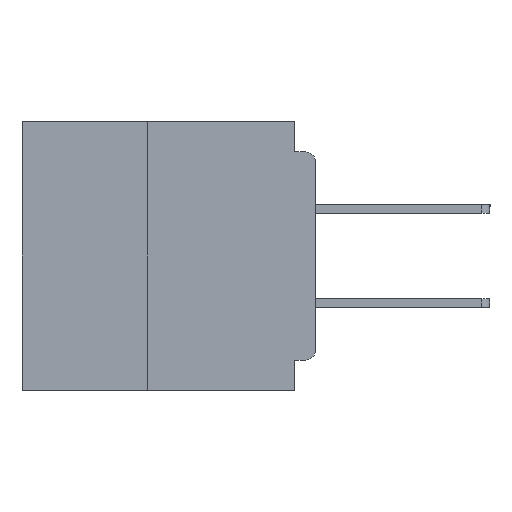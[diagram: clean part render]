
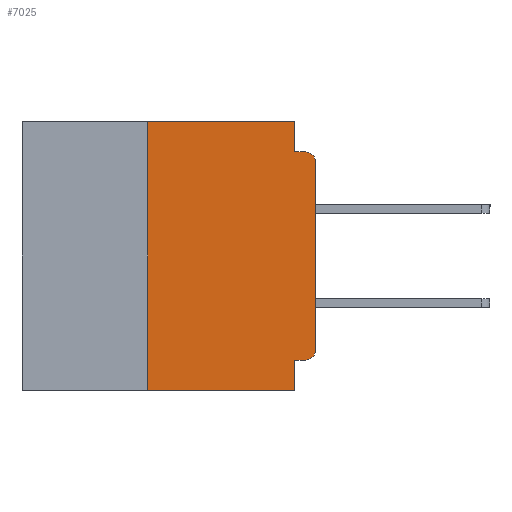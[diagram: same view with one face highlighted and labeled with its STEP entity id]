
A CAD part, left-side view. The second image highlights one B-rep face of the part: STEP entity #7025.
In plain terms, the highlighted planar face has unit normal (-1, 0, 0).
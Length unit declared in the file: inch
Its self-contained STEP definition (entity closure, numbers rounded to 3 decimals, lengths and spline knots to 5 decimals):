
#572 = CARTESIAN_POINT ( 'NONE',  ( 0., 0.25, -0.4 ) ) ;
#629 = VERTEX_POINT ( 'NONE', #41840 ) ;
#708 = EDGE_CURVE ( 'NONE', #14228, #19396, #25253, .T. ) ;
#2983 = VERTEX_POINT ( 'NONE', #5823 ) ;
#3160 = ORIENTED_EDGE ( 'NONE', *, *, #9187, .F. ) ;
#3955 = VECTOR ( 'NONE', #57200, 39.37008 ) ;
#4021 = CARTESIAN_POINT ( 'NONE',  ( 0., 0.031, 0. ) ) ;
#4068 = LINE ( 'NONE', #31584, #53552 ) ;
#4094 = FACE_OUTER_BOUND ( 'NONE', #14544, .T. ) ;
#4369 = DIRECTION ( 'NONE',  ( 0., 0., -1. ) ) ;
#4866 = CARTESIAN_POINT ( 'NONE',  ( 0., 0.25, 0. ) ) ;
#4978 = CARTESIAN_POINT ( 'NONE',  ( 0., 0.031, -0.4 ) ) ;
#5363 = ORIENTED_EDGE ( 'NONE', *, *, #708, .F. ) ;
#5823 = CARTESIAN_POINT ( 'NONE',  ( 0., 0.031, 0. ) ) ;
#7025 = ADVANCED_FACE ( 'NONE', ( #4094 ), #35545, .F. ) ;
#7192 = ORIENTED_EDGE ( 'NONE', *, *, #42871, .F. ) ;
#7927 = EDGE_CURVE ( 'NONE', #8041, #629, #40062, .T. ) ;
#8041 = VERTEX_POINT ( 'NONE', #54404 ) ;
#8421 = AXIS2_PLACEMENT_3D ( 'NONE', #27969, #61461, #32789 ) ;
#9187 = EDGE_CURVE ( 'NONE', #36276, #23664, #55641, .T. ) ;
#9914 = CARTESIAN_POINT ( 'NONE',  ( 0., 0.015, -0.045 ) ) ;
#10150 = EDGE_CURVE ( 'NONE', #22736, #23664, #25517, .T. ) ;
#10203 = DIRECTION ( 'NONE',  ( 0., 0., 1. ) ) ;
#11005 = VECTOR ( 'NONE', #36324, 39.37008 ) ;
#11325 = ORIENTED_EDGE ( 'NONE', *, *, #7927, .T. ) ;
#13453 = VERTEX_POINT ( 'NONE', #34746 ) ;
#14228 = VERTEX_POINT ( 'NONE', #31449 ) ;
#14544 = EDGE_LOOP ( 'NONE', ( #39849, #36387, #3160, #15448, #15174, #7192, #41543, #5363, #51667, #11325 ) ) ;
#15174 = ORIENTED_EDGE ( 'NONE', *, *, #57435, .F. ) ;
#15314 = CARTESIAN_POINT ( 'NONE',  ( 0., 0., -0.045 ) ) ;
#15448 = ORIENTED_EDGE ( 'NONE', *, *, #52084, .F. ) ;
#17462 = LINE ( 'NONE', #572, #27146 ) ;
#18926 = CARTESIAN_POINT ( 'NONE',  ( 0., 0., 0. ) ) ;
#19396 = VERTEX_POINT ( 'NONE', #33684 ) ;
#20051 = DIRECTION ( 'NONE',  ( -1., 0., 0. ) ) ;
#21300 = DIRECTION ( 'NONE',  ( 0., 0., -1. ) ) ;
#22736 = VERTEX_POINT ( 'NONE', #36203 ) ;
#23620 = LINE ( 'NONE', #43675, #58829 ) ;
#23664 = VERTEX_POINT ( 'NONE', #9914 ) ;
#23716 = LINE ( 'NONE', #55398, #11005 ) ;
#25253 = LINE ( 'NONE', #4978, #49271 ) ;
#25517 = CIRCLE ( 'NONE', #8421, 0.015 ) ;
#27146 = VECTOR ( 'NONE', #10203, 39.37008 ) ;
#27969 = CARTESIAN_POINT ( 'NONE',  ( 0., 0.015, -0.06 ) ) ;
#29386 = EDGE_CURVE ( 'NONE', #13453, #19396, #23620, .T. ) ;
#30171 = VECTOR ( 'NONE', #37528, 39.37008 ) ;
#30730 = CARTESIAN_POINT ( 'NONE',  ( 0., 0.437, 0. ) ) ;
#30935 = LINE ( 'NONE', #18926, #3955 ) ;
#31449 = CARTESIAN_POINT ( 'NONE',  ( 0., 0.031, -0.355 ) ) ;
#31584 = CARTESIAN_POINT ( 'NONE',  ( 0., 0., -0.355 ) ) ;
#31733 = VERTEX_POINT ( 'NONE', #4866 ) ;
#32789 = DIRECTION ( 'NONE',  ( 0., 0., -1. ) ) ;
#33684 = CARTESIAN_POINT ( 'NONE',  ( 0., 0.031, -0.4 ) ) ;
#34746 = CARTESIAN_POINT ( 'NONE',  ( 0., 0.25, -0.4 ) ) ;
#35545 = PLANE ( 'NONE',  #53681 ) ;
#36203 = CARTESIAN_POINT ( 'NONE',  ( 0., 0., -0.06 ) ) ;
#36276 = VERTEX_POINT ( 'NONE', #51579 ) ;
#36324 = DIRECTION ( 'NONE',  ( 0., -1., 0. ) ) ;
#36387 = ORIENTED_EDGE ( 'NONE', *, *, #10150, .T. ) ;
#37528 = DIRECTION ( 'NONE',  ( 0., 0., -1. ) ) ;
#39849 = ORIENTED_EDGE ( 'NONE', *, *, #59602, .T. ) ;
#40062 = CIRCLE ( 'NONE', #40445, 0.015 ) ;
#40445 = AXIS2_PLACEMENT_3D ( 'NONE', #48772, #20051, #53590 ) ;
#40973 = DIRECTION ( 'NONE',  ( 0., 1., 0. ) ) ;
#41543 = ORIENTED_EDGE ( 'NONE', *, *, #29386, .T. ) ;
#41840 = CARTESIAN_POINT ( 'NONE',  ( 0., 0., -0.34 ) ) ;
#42871 = EDGE_CURVE ( 'NONE', #13453, #31733, #17462, .T. ) ;
#42882 = VECTOR ( 'NONE', #53443, 39.37008 ) ;
#42894 = LINE ( 'NONE', #4021, #30171 ) ;
#43675 = CARTESIAN_POINT ( 'NONE',  ( 0., 0.437, -0.4 ) ) ;
#48524 = DIRECTION ( 'NONE',  ( 0., -1., 0. ) ) ;
#48772 = CARTESIAN_POINT ( 'NONE',  ( 0., 0.015, -0.34 ) ) ;
#49271 = VECTOR ( 'NONE', #4369, 39.37008 ) ;
#50030 = DIRECTION ( 'NONE',  ( 1., 0., 0. ) ) ;
#51579 = CARTESIAN_POINT ( 'NONE',  ( 0., 0.031, -0.045 ) ) ;
#51667 = ORIENTED_EDGE ( 'NONE', *, *, #58747, .F. ) ;
#52084 = EDGE_CURVE ( 'NONE', #2983, #36276, #42894, .T. ) ;
#53443 = DIRECTION ( 'NONE',  ( 0., -1., 0. ) ) ;
#53552 = VECTOR ( 'NONE', #40973, 39.37008 ) ;
#53590 = DIRECTION ( 'NONE',  ( 0., 0., -1. ) ) ;
#53681 = AXIS2_PLACEMENT_3D ( 'NONE', #30730, #50030, #21300 ) ;
#54404 = CARTESIAN_POINT ( 'NONE',  ( 0., 0.015, -0.355 ) ) ;
#55398 = CARTESIAN_POINT ( 'NONE',  ( 0., 0.437, 0. ) ) ;
#55641 = LINE ( 'NONE', #15314, #42882 ) ;
#57200 = DIRECTION ( 'NONE',  ( 0., 0., 1. ) ) ;
#57435 = EDGE_CURVE ( 'NONE', #31733, #2983, #23716, .T. ) ;
#58747 = EDGE_CURVE ( 'NONE', #8041, #14228, #4068, .T. ) ;
#58829 = VECTOR ( 'NONE', #48524, 39.37008 ) ;
#59602 = EDGE_CURVE ( 'NONE', #629, #22736, #30935, .T. ) ;
#61461 = DIRECTION ( 'NONE',  ( -1., 0., 0. ) ) ;
